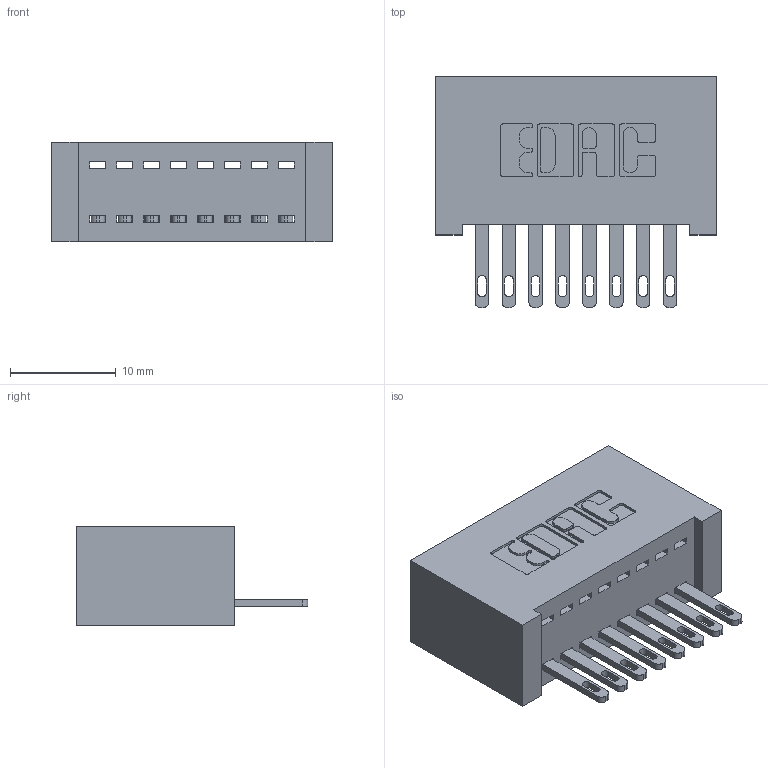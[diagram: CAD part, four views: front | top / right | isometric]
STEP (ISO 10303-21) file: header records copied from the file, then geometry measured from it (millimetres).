
FILE_DESCRIPTION (( 'STEP AP203' ), '1' );
FILE_NAME ('892-008-500-101.STEP', '2020-09-21T12:36:29', ( '' ), ( '' ), 'SwSTEP 2.0', 'SolidWorks 2020', '' );
FILE_SCHEMA (( 'CONFIG_CONTROL_DESIGN' ));
Length unit declared in the file: inch
Products named in the file (3): 345-292-001_345-293-100; 892-008-500-101; 842 Part_Lugless
Assembly tree (9 placements, depth 2):
  892-008-500-101
    842 Part_Lugless
    345-292-001_345-293-100  x8
Bounding box: 26.57 x 21.85 x 9.4 mm (x, y, z)
Volume: 2618.2 mm3; surface area: 3548.9 mm2
Topology: 9 solids, 9 shells, 534 faces, 1619 edges, 1078 vertices
Faces by surface type: plane 350, cylinder 184
Entity records: 8809 total; most frequent: CARTESIAN_POINT 1530, ORIENTED_EDGE 1474, DIRECTION 1353, EDGE_CURVE 737, VECTOR 613, LINE 613, VERTEX_POINT 490, AXIS2_PLACEMENT_3D 370
